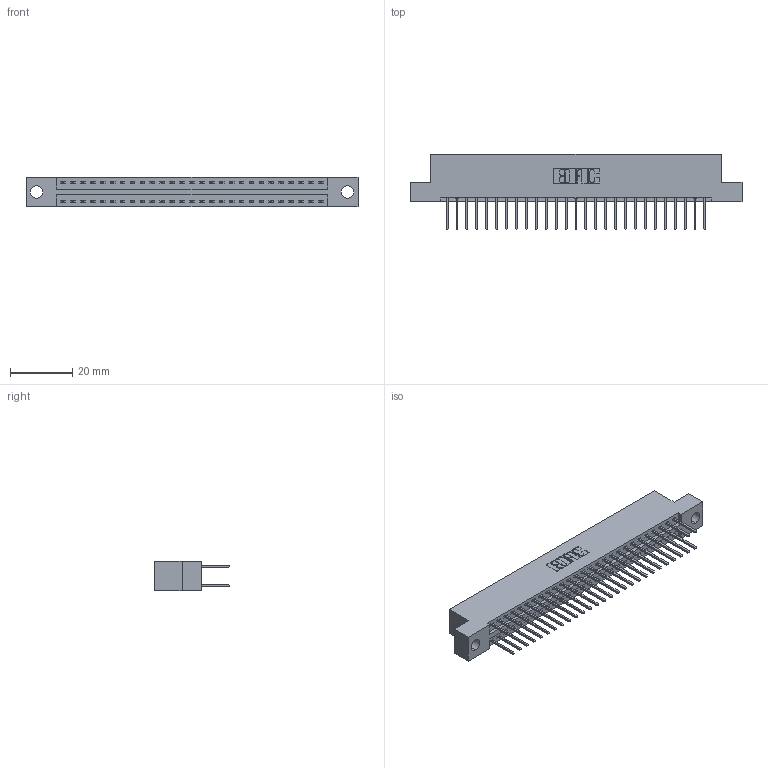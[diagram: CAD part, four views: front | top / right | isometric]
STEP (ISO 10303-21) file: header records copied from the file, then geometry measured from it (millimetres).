
FILE_DESCRIPTION (( 'STEP AP203' ), '1' );
FILE_NAME ('346-054-526-204.STEP', '2022-05-21T03:13:59', ( '' ), ( '' ), 'SwSTEP 2.0', 'SolidWorks 2020', '' );
FILE_SCHEMA (( 'CONFIG_CONTROL_DESIGN' ));
Length unit declared in the file: inch
Products named in the file (3): 345-292-001_345-293-126; 346 Part_Flush Mounting Lugs - 0.156 Dia-TH; 346-054-526-204
Assembly tree (55 placements, depth 2):
  346-054-526-204
    346 Part_Flush Mounting Lugs - 0.156 Dia-TH
    345-292-001_345-293-126  x54
Bounding box: 106.3 x 24.13 x 9.4 mm (x, y, z)
Volume: 10231.6 mm3; surface area: 14072.5 mm2
Topology: 55 solids, 55 shells, 2944 faces, 8735 edges, 5750 vertices
Faces by surface type: plane 1980, cylinder 964
Entity records: 20077 total; most frequent: CARTESIAN_POINT 3334, ORIENTED_EDGE 3266, DIRECTION 2989, EDGE_CURVE 1633, VECTOR 1393, LINE 1393, VERTEX_POINT 1086, AXIS2_PLACEMENT_3D 798
